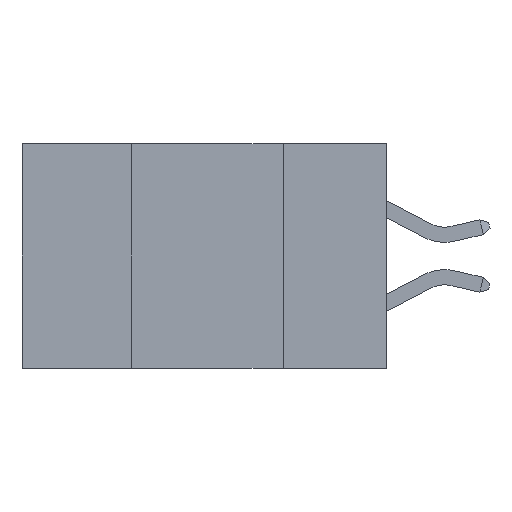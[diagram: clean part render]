
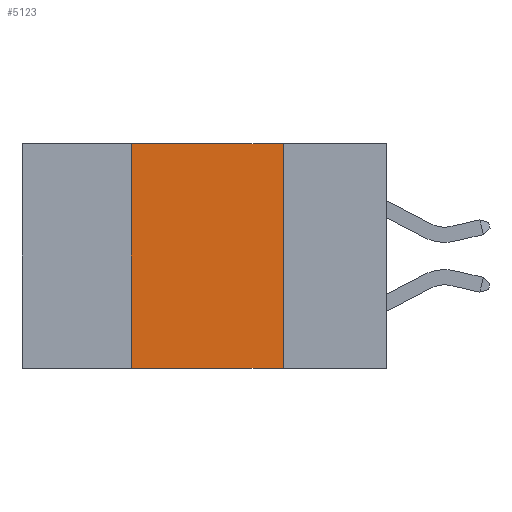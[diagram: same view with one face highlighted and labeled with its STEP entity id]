
A CAD part, left-side view. The second image highlights one B-rep face of the part: STEP entity #5123.
In plain terms, the highlighted planar face has unit normal (-1, 0, 0).
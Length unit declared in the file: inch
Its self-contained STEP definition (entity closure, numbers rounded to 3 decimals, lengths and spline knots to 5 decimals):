
#106 = FACE_OUTER_BOUND ( 'NONE', #2061, .T. ) ;
#196 = CARTESIAN_POINT ( 'NONE',  ( 0., 0.17, 0. ) ) ;
#935 = EDGE_CURVE ( 'NONE', #5591, #8336, #9420, .T. ) ;
#950 = ORIENTED_EDGE ( 'NONE', *, *, #3072, .F. ) ;
#1096 = DIRECTION ( 'NONE',  ( 0., -1., 0. ) ) ;
#1245 = DIRECTION ( 'NONE',  ( 0., 0., -1. ) ) ;
#1408 = ORIENTED_EDGE ( 'NONE', *, *, #6018, .F. ) ;
#2044 = CARTESIAN_POINT ( 'NONE',  ( 0., 0.6, -0.37 ) ) ;
#2061 = EDGE_LOOP ( 'NONE', ( #1408, #950, #5675, #5572 ) ) ;
#2576 = VERTEX_POINT ( 'NONE', #196 ) ;
#3072 = EDGE_CURVE ( 'NONE', #8304, #2576, #4709, .T. ) ;
#3718 = CARTESIAN_POINT ( 'NONE',  ( 0., 0.17, -0.37 ) ) ;
#3720 = DIRECTION ( 'NONE',  ( 0., 0., -1. ) ) ;
#3738 = DIRECTION ( 'NONE',  ( 1., 0., 0. ) ) ;
#3808 = CARTESIAN_POINT ( 'NONE',  ( 0., 0.6, 0. ) ) ;
#3818 = PLANE ( 'NONE',  #9515 ) ;
#4468 = VECTOR ( 'NONE', #4566, 39.37008 ) ;
#4566 = DIRECTION ( 'NONE',  ( 0., -1., 0. ) ) ;
#4577 = VECTOR ( 'NONE', #1245, 39.37008 ) ;
#4709 = LINE ( 'NONE', #9352, #4468 ) ;
#5123 = ADVANCED_FACE ( 'NONE', ( #106 ), #3818, .F. ) ;
#5538 = DIRECTION ( 'NONE',  ( 0., 0., 1. ) ) ;
#5572 = ORIENTED_EDGE ( 'NONE', *, *, #935, .T. ) ;
#5591 = VERTEX_POINT ( 'NONE', #6483 ) ;
#5675 = ORIENTED_EDGE ( 'NONE', *, *, #8587, .F. ) ;
#6018 = EDGE_CURVE ( 'NONE', #2576, #8336, #6599, .T. ) ;
#6060 = CARTESIAN_POINT ( 'NONE',  ( 0., 0.17, 0. ) ) ;
#6483 = CARTESIAN_POINT ( 'NONE',  ( 0., 0.42, -0.37 ) ) ;
#6599 = LINE ( 'NONE', #6060, #4577 ) ;
#6998 = VECTOR ( 'NONE', #1096, 39.37008 ) ;
#7759 = LINE ( 'NONE', #7825, #9443 ) ;
#7825 = CARTESIAN_POINT ( 'NONE',  ( 0., 0.42, 0. ) ) ;
#8304 = VERTEX_POINT ( 'NONE', #8986 ) ;
#8336 = VERTEX_POINT ( 'NONE', #3718 ) ;
#8587 = EDGE_CURVE ( 'NONE', #5591, #8304, #7759, .T. ) ;
#8986 = CARTESIAN_POINT ( 'NONE',  ( 0., 0.42, 0. ) ) ;
#9352 = CARTESIAN_POINT ( 'NONE',  ( 0., 0.6, 0. ) ) ;
#9420 = LINE ( 'NONE', #2044, #6998 ) ;
#9443 = VECTOR ( 'NONE', #5538, 39.37008 ) ;
#9515 = AXIS2_PLACEMENT_3D ( 'NONE', #3808, #3738, #3720 ) ;
